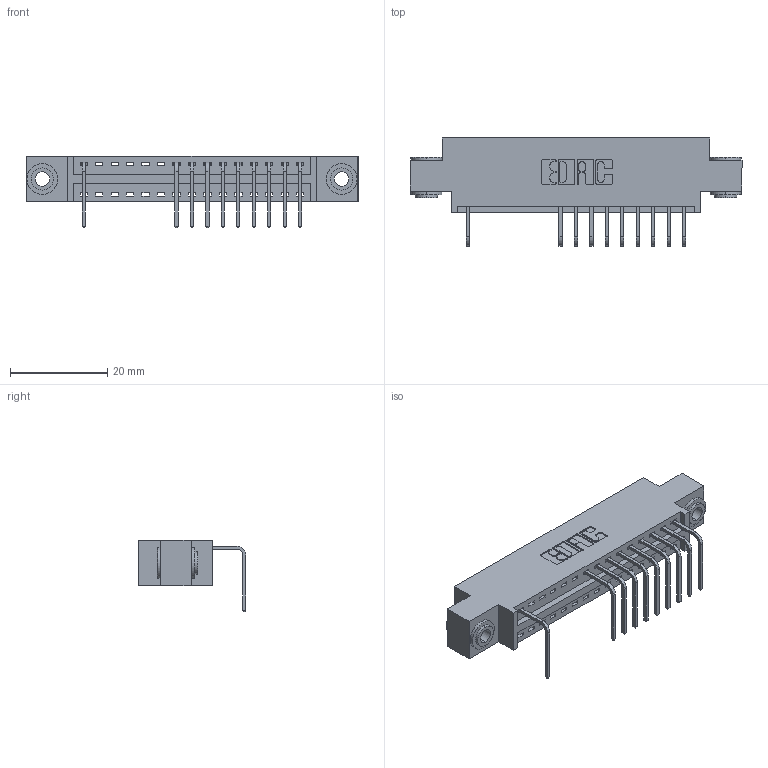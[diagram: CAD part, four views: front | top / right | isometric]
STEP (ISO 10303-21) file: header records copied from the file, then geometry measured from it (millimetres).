
FILE_DESCRIPTION (( 'STEP AP203' ), '1' );
FILE_NAME ('346-015-558-603.STEP', '2018-08-20T03:07:12', ( '' ), ( '' ), 'SwSTEP 2.0', 'SolidWorks 2016', '' );
FILE_SCHEMA (( 'CONFIG_CONTROL_DESIGN' ));
Length unit declared in the file: inch
Products named in the file (4): 345-250-002_345-250-002-102; 346-015-558-603; 346 Part_0.170 Offset - 0.156 Dia-TH; 345-292-001_558 Tail - 2
Assembly tree (13 placements, depth 2):
  346-015-558-603
    346 Part_0.170 Offset - 0.156 Dia-TH
    345-292-001_558 Tail - 2  x10
    345-250-002_345-250-002-102  x2
Bounding box: 68.2 x 22.16 x 14.73 mm (x, y, z)
Volume: 6183.1 mm3; surface area: 7707.3 mm2
Topology: 13 solids, 13 shells, 824 faces, 2447 edges, 1614 vertices
Faces by surface type: plane 560, cylinder 256, cone 8
Entity records: 13650 total; most frequent: CARTESIAN_POINT 2351, ORIENTED_EDGE 2298, DIRECTION 2131, EDGE_CURVE 1149, VECTOR 933, LINE 933, VERTEX_POINT 762, AXIS2_PLACEMENT_3D 599
